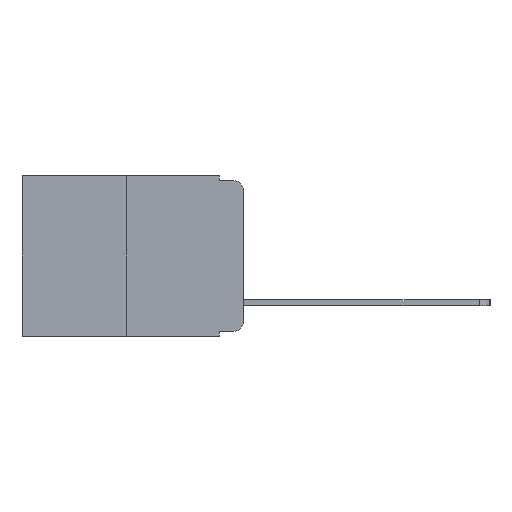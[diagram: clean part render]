
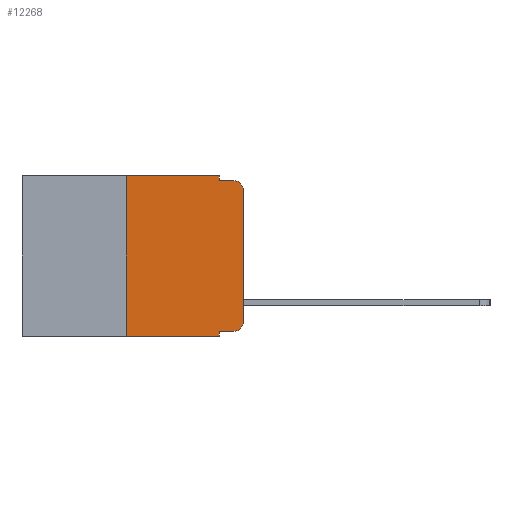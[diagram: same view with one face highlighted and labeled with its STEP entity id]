
A CAD part, left-side view. The second image highlights one B-rep face of the part: STEP entity #12268.
In plain terms, the highlighted planar face has unit normal (-1, 0, 0).
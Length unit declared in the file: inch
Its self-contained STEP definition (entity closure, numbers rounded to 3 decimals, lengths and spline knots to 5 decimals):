
#142 = VERTEX_POINT ( 'NONE', #12996 ) ;
#149 = CARTESIAN_POINT ( 'NONE',  ( 0., 0.25, 0. ) ) ;
#410 = EDGE_CURVE ( 'NONE', #5672, #13253, #11465, .T. ) ;
#596 = DIRECTION ( 'NONE',  ( 0., -1., 0. ) ) ;
#795 = DIRECTION ( 'NONE',  ( -1., 0., 0. ) ) ;
#997 = CARTESIAN_POINT ( 'NONE',  ( 0., 0.051, 0. ) ) ;
#1165 = VERTEX_POINT ( 'NONE', #3533 ) ;
#1533 = CARTESIAN_POINT ( 'NONE',  ( 0., 0., -0.313 ) ) ;
#1911 = VECTOR ( 'NONE', #2552, 39.37008 ) ;
#2173 = VECTOR ( 'NONE', #596, 39.37008 ) ;
#2414 = CARTESIAN_POINT ( 'NONE',  ( 0., 0.473, 0. ) ) ;
#2533 = EDGE_CURVE ( 'NONE', #14117, #15671, #4202, .T. ) ;
#2552 = DIRECTION ( 'NONE',  ( 0., -1., 0. ) ) ;
#2585 = DIRECTION ( 'NONE',  ( 0., 0., -1. ) ) ;
#2799 = CARTESIAN_POINT ( 'NONE',  ( 0., 0.02, -0.03 ) ) ;
#3452 = VECTOR ( 'NONE', #2585, 39.37008 ) ;
#3533 = CARTESIAN_POINT ( 'NONE',  ( 0., 0.02, -0.01 ) ) ;
#3626 = ORIENTED_EDGE ( 'NONE', *, *, #10811, .T. ) ;
#4035 = DIRECTION ( 'NONE',  ( 0., -1., 0. ) ) ;
#4202 = LINE ( 'NONE', #4794, #11864 ) ;
#4352 = DIRECTION ( 'NONE',  ( 0., 0., -1. ) ) ;
#4539 = CARTESIAN_POINT ( 'NONE',  ( 0., 0., -0.03 ) ) ;
#4605 = EDGE_CURVE ( 'NONE', #142, #14104, #15440, .T. ) ;
#4794 = CARTESIAN_POINT ( 'NONE',  ( 0., 0.25, 0. ) ) ;
#4862 = EDGE_LOOP ( 'NONE', ( #3626, #15648, #16964, #13383, #10857, #15594, #13175, #11573, #15450, #15247 ) ) ;
#5118 = CIRCLE ( 'NONE', #9103, 0.02 ) ;
#5672 = VERTEX_POINT ( 'NONE', #15555 ) ;
#5710 = EDGE_CURVE ( 'NONE', #14104, #1165, #13845, .T. ) ;
#5728 = CARTESIAN_POINT ( 'NONE',  ( 0., 0.051, -0.333 ) ) ;
#6776 = EDGE_CURVE ( 'NONE', #16323, #1165, #11300, .T. ) ;
#7108 = CARTESIAN_POINT ( 'NONE',  ( 0., 0.25, -0.343 ) ) ;
#7499 = VECTOR ( 'NONE', #8958, 39.37008 ) ;
#7513 = VECTOR ( 'NONE', #13782, 39.37008 ) ;
#7639 = DIRECTION ( 'NONE',  ( 1., 0., 0. ) ) ;
#8342 = VERTEX_POINT ( 'NONE', #1533 ) ;
#8509 = CARTESIAN_POINT ( 'NONE',  ( 0., 0.02, -0.333 ) ) ;
#8958 = DIRECTION ( 'NONE',  ( 0., 0., -1. ) ) ;
#9103 = AXIS2_PLACEMENT_3D ( 'NONE', #10084, #795, #11588 ) ;
#9258 = VECTOR ( 'NONE', #4035, 39.37008 ) ;
#9741 = CARTESIAN_POINT ( 'NONE',  ( 0., 0.051, 0. ) ) ;
#10084 = CARTESIAN_POINT ( 'NONE',  ( 0., 0.02, -0.313 ) ) ;
#10811 = EDGE_CURVE ( 'NONE', #8342, #16323, #15750, .T. ) ;
#10857 = ORIENTED_EDGE ( 'NONE', *, *, #14628, .F. ) ;
#11300 = CIRCLE ( 'NONE', #18281, 0.02 ) ;
#11325 = EDGE_CURVE ( 'NONE', #14117, #13253, #11480, .T. ) ;
#11465 = LINE ( 'NONE', #9741, #7499 ) ;
#11480 = LINE ( 'NONE', #12319, #7513 ) ;
#11573 = ORIENTED_EDGE ( 'NONE', *, *, #410, .F. ) ;
#11588 = DIRECTION ( 'NONE',  ( 0., 0., -1. ) ) ;
#11864 = VECTOR ( 'NONE', #15579, 39.37008 ) ;
#12268 = ADVANCED_FACE ( 'NONE', ( #15473 ), #19134, .F. ) ;
#12319 = CARTESIAN_POINT ( 'NONE',  ( 0., 0.473, -0.343 ) ) ;
#12647 = VERTEX_POINT ( 'NONE', #8509 ) ;
#12996 = CARTESIAN_POINT ( 'NONE',  ( 0., 0.051, 0. ) ) ;
#13175 = ORIENTED_EDGE ( 'NONE', *, *, #11325, .T. ) ;
#13253 = VERTEX_POINT ( 'NONE', #14355 ) ;
#13347 = VECTOR ( 'NONE', #16359, 39.37008 ) ;
#13383 = ORIENTED_EDGE ( 'NONE', *, *, #4605, .F. ) ;
#13460 = DIRECTION ( 'NONE',  ( -1., 0., 0. ) ) ;
#13657 = LINE ( 'NONE', #2414, #9258 ) ;
#13782 = DIRECTION ( 'NONE',  ( 0., -1., 0. ) ) ;
#13845 = LINE ( 'NONE', #15729, #2173 ) ;
#14104 = VERTEX_POINT ( 'NONE', #15850 ) ;
#14117 = VERTEX_POINT ( 'NONE', #7108 ) ;
#14355 = CARTESIAN_POINT ( 'NONE',  ( 0., 0.051, -0.343 ) ) ;
#14628 = EDGE_CURVE ( 'NONE', #15671, #142, #13657, .T. ) ;
#14954 = CARTESIAN_POINT ( 'NONE',  ( 0., 0., 0. ) ) ;
#14962 = CARTESIAN_POINT ( 'NONE',  ( 0., 0.473, 0. ) ) ;
#15196 = AXIS2_PLACEMENT_3D ( 'NONE', #14962, #7639, #17771 ) ;
#15247 = ORIENTED_EDGE ( 'NONE', *, *, #15979, .T. ) ;
#15440 = LINE ( 'NONE', #997, #3452 ) ;
#15450 = ORIENTED_EDGE ( 'NONE', *, *, #16921, .T. ) ;
#15473 = FACE_OUTER_BOUND ( 'NONE', #4862, .T. ) ;
#15555 = CARTESIAN_POINT ( 'NONE',  ( 0., 0.051, -0.333 ) ) ;
#15579 = DIRECTION ( 'NONE',  ( 0., 0., 1. ) ) ;
#15594 = ORIENTED_EDGE ( 'NONE', *, *, #2533, .F. ) ;
#15648 = ORIENTED_EDGE ( 'NONE', *, *, #6776, .T. ) ;
#15671 = VERTEX_POINT ( 'NONE', #149 ) ;
#15729 = CARTESIAN_POINT ( 'NONE',  ( 0., 0.051, -0.01 ) ) ;
#15750 = LINE ( 'NONE', #14954, #13347 ) ;
#15850 = CARTESIAN_POINT ( 'NONE',  ( 0., 0.051, -0.01 ) ) ;
#15979 = EDGE_CURVE ( 'NONE', #12647, #8342, #5118, .T. ) ;
#16323 = VERTEX_POINT ( 'NONE', #4539 ) ;
#16359 = DIRECTION ( 'NONE',  ( 0., 0., 1. ) ) ;
#16921 = EDGE_CURVE ( 'NONE', #5672, #12647, #17769, .T. ) ;
#16964 = ORIENTED_EDGE ( 'NONE', *, *, #5710, .F. ) ;
#17769 = LINE ( 'NONE', #5728, #1911 ) ;
#17771 = DIRECTION ( 'NONE',  ( 0., 0., -1. ) ) ;
#18281 = AXIS2_PLACEMENT_3D ( 'NONE', #2799, #13460, #4352 ) ;
#19134 = PLANE ( 'NONE',  #15196 ) ;
